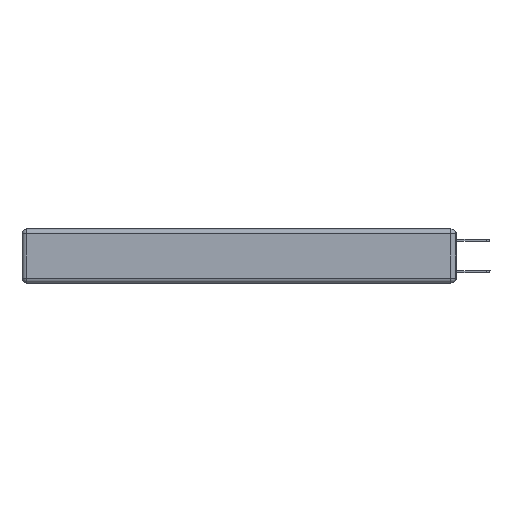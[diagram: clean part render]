
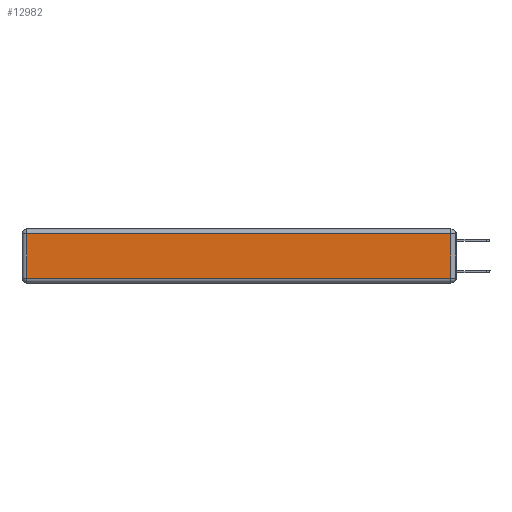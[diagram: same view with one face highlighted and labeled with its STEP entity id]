
A CAD part, left-side view. The second image highlights one B-rep face of the part: STEP entity #12982.
In plain terms, the highlighted planar face has unit normal (-1, 0, 0).
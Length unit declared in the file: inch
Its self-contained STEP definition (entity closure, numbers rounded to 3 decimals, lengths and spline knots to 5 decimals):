
#1014 = DIRECTION ( 'NONE',  ( 0., 0., 1. ) ) ;
#1133 = VECTOR ( 'NONE', #15816, 39.37008 ) ;
#1367 = DIRECTION ( 'NONE',  ( 0., 1., 0. ) ) ;
#1518 = VERTEX_POINT ( 'NONE', #7741 ) ;
#1617 = EDGE_CURVE ( 'NONE', #1518, #6798, #3607, .T. ) ;
#1891 = VECTOR ( 'NONE', #1367, 39.37008 ) ;
#2476 = ORIENTED_EDGE ( 'NONE', *, *, #1617, .T. ) ;
#2816 = LINE ( 'NONE', #15140, #1891 ) ;
#2918 = DIRECTION ( 'NONE',  ( -1., 0., 0. ) ) ;
#3025 = CARTESIAN_POINT ( 'NONE',  ( 0., 0.03, -0.313 ) ) ;
#3127 = CARTESIAN_POINT ( 'NONE',  ( 0., 2.72, -0.343 ) ) ;
#3607 = LINE ( 'NONE', #16102, #12100 ) ;
#4966 = VERTEX_POINT ( 'NONE', #7826 ) ;
#6482 = DIRECTION ( 'NONE',  ( 0., -1., 0. ) ) ;
#6798 = VERTEX_POINT ( 'NONE', #3025 ) ;
#6974 = DIRECTION ( 'NONE',  ( 0., 0., 1. ) ) ;
#7731 = CARTESIAN_POINT ( 'NONE',  ( 0., 0.03, -0.03 ) ) ;
#7741 = CARTESIAN_POINT ( 'NONE',  ( 0., 2.72, -0.313 ) ) ;
#7826 = CARTESIAN_POINT ( 'NONE',  ( 0., 2.72, -0.03 ) ) ;
#7859 = LINE ( 'NONE', #13398, #17723 ) ;
#8151 = EDGE_CURVE ( 'NONE', #6798, #9052, #7859, .T. ) ;
#8205 = EDGE_LOOP ( 'NONE', ( #2476, #15068, #10129, #11265 ) ) ;
#9052 = VERTEX_POINT ( 'NONE', #7731 ) ;
#9774 = PLANE ( 'NONE',  #12910 ) ;
#10129 = ORIENTED_EDGE ( 'NONE', *, *, #11469, .T. ) ;
#11265 = ORIENTED_EDGE ( 'NONE', *, *, #16940, .T. ) ;
#11469 = EDGE_CURVE ( 'NONE', #9052, #4966, #2816, .T. ) ;
#11622 = LINE ( 'NONE', #3127, #1133 ) ;
#12100 = VECTOR ( 'NONE', #6482, 39.37008 ) ;
#12910 = AXIS2_PLACEMENT_3D ( 'NONE', #16781, #2918, #6974 ) ;
#12982 = ADVANCED_FACE ( 'NONE', ( #15328 ), #9774, .T. ) ;
#13398 = CARTESIAN_POINT ( 'NONE',  ( 0., 0.03, -0.343 ) ) ;
#15068 = ORIENTED_EDGE ( 'NONE', *, *, #8151, .T. ) ;
#15140 = CARTESIAN_POINT ( 'NONE',  ( 0., 2.75, -0.03 ) ) ;
#15328 = FACE_OUTER_BOUND ( 'NONE', #8205, .T. ) ;
#15816 = DIRECTION ( 'NONE',  ( 0., 0., -1. ) ) ;
#16102 = CARTESIAN_POINT ( 'NONE',  ( 0., 0., -0.313 ) ) ;
#16781 = CARTESIAN_POINT ( 'NONE',  ( 0., 0., -0.343 ) ) ;
#16940 = EDGE_CURVE ( 'NONE', #4966, #1518, #11622, .T. ) ;
#17723 = VECTOR ( 'NONE', #1014, 39.37008 ) ;
